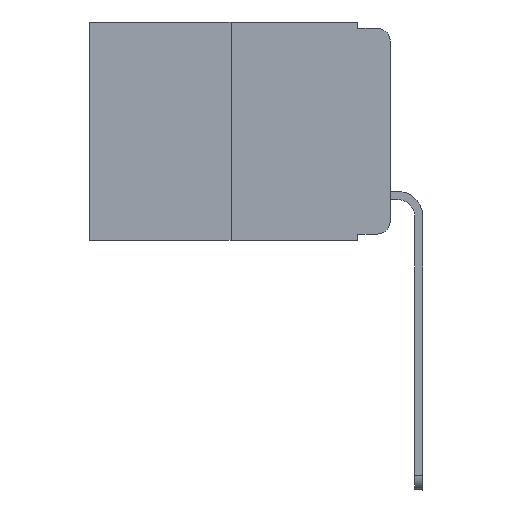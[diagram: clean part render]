
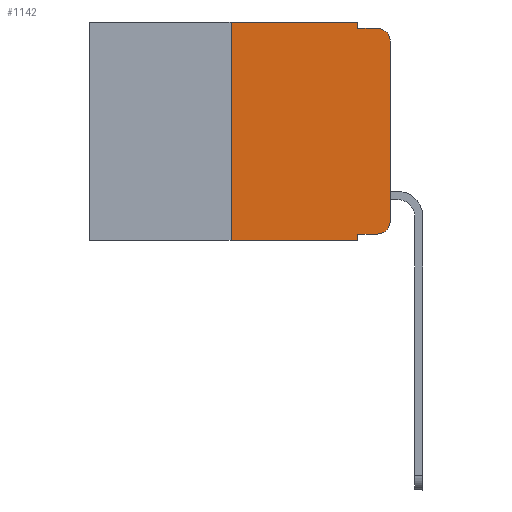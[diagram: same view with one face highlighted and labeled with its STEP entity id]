
A CAD part, left-side view. The second image highlights one B-rep face of the part: STEP entity #1142.
In plain terms, the highlighted planar face has unit normal (-1, 0, 0).
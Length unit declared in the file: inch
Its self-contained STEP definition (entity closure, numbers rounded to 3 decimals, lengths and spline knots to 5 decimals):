
#118 = LINE ( 'NONE', #17399, #14100 ) ;
#137 = CARTESIAN_POINT ( 'NONE',  ( 0., 0.25, 0. ) ) ;
#210 = VECTOR ( 'NONE', #14992, 39.37008 ) ;
#268 = CIRCLE ( 'NONE', #9839, 0.02 ) ;
#355 = DIRECTION ( 'NONE',  ( 0., 0., -1. ) ) ;
#669 = EDGE_CURVE ( 'NONE', #5832, #14060, #118, .T. ) ;
#944 = CARTESIAN_POINT ( 'NONE',  ( 0., 0.25, -0.343 ) ) ;
#1142 = ADVANCED_FACE ( 'NONE', ( #17478 ), #5065, .F. ) ;
#1300 = VERTEX_POINT ( 'NONE', #16242 ) ;
#2220 = CARTESIAN_POINT ( 'NONE',  ( 0., 0.051, 0. ) ) ;
#2387 = ORIENTED_EDGE ( 'NONE', *, *, #20250, .F. ) ;
#3451 = ORIENTED_EDGE ( 'NONE', *, *, #10100, .F. ) ;
#3879 = EDGE_LOOP ( 'NONE', ( #17752, #15207, #17142, #3451, #15063, #2387, #17645, #16792, #17777, #17153 ) ) ;
#3902 = VECTOR ( 'NONE', #18713, 39.37008 ) ;
#3994 = CARTESIAN_POINT ( 'NONE',  ( 0., 0., -0.313 ) ) ;
#4027 = VERTEX_POINT ( 'NONE', #12173 ) ;
#4070 = LINE ( 'NONE', #15347, #5604 ) ;
#4444 = DIRECTION ( 'NONE',  ( -1., 0., 0. ) ) ;
#5065 = PLANE ( 'NONE',  #8002 ) ;
#5604 = VECTOR ( 'NONE', #8839, 39.37008 ) ;
#5832 = VERTEX_POINT ( 'NONE', #19000 ) ;
#6149 = CARTESIAN_POINT ( 'NONE',  ( 0., 0.02, -0.01 ) ) ;
#6307 = EDGE_CURVE ( 'NONE', #10307, #6653, #14230, .T. ) ;
#6369 = CARTESIAN_POINT ( 'NONE',  ( 0., 0., 0. ) ) ;
#6458 = DIRECTION ( 'NONE',  ( 0., 0., 1. ) ) ;
#6544 = DIRECTION ( 'NONE',  ( 0., -1., 0. ) ) ;
#6653 = VERTEX_POINT ( 'NONE', #20296 ) ;
#6785 = AXIS2_PLACEMENT_3D ( 'NONE', #16962, #4444, #19852 ) ;
#6885 = LINE ( 'NONE', #2220, #15857 ) ;
#6969 = VERTEX_POINT ( 'NONE', #7750 ) ;
#6989 = DIRECTION ( 'NONE',  ( -1., 0., 0. ) ) ;
#7430 = VECTOR ( 'NONE', #15981, 39.37008 ) ;
#7750 = CARTESIAN_POINT ( 'NONE',  ( 0., 0.25, 0. ) ) ;
#7893 = EDGE_CURVE ( 'NONE', #6969, #1300, #4070, .T. ) ;
#8002 = AXIS2_PLACEMENT_3D ( 'NONE', #9623, #14178, #19233 ) ;
#8839 = DIRECTION ( 'NONE',  ( 0., -1., 0. ) ) ;
#8868 = EDGE_CURVE ( 'NONE', #11155, #14629, #9200, .T. ) ;
#8897 = EDGE_CURVE ( 'NONE', #11449, #10307, #268, .T. ) ;
#9062 = VECTOR ( 'NONE', #6458, 39.37008 ) ;
#9200 = LINE ( 'NONE', #12411, #3902 ) ;
#9623 = CARTESIAN_POINT ( 'NONE',  ( 0., 0.473, 0. ) ) ;
#9724 = CARTESIAN_POINT ( 'NONE',  ( 0., 0.02, -0.333 ) ) ;
#9839 = AXIS2_PLACEMENT_3D ( 'NONE', #18035, #6989, #14740 ) ;
#10100 = EDGE_CURVE ( 'NONE', #1300, #5832, #11665, .T. ) ;
#10307 = VERTEX_POINT ( 'NONE', #3994 ) ;
#10661 = EDGE_CURVE ( 'NONE', #4027, #14629, #6885, .T. ) ;
#11155 = VERTEX_POINT ( 'NONE', #944 ) ;
#11379 = CARTESIAN_POINT ( 'NONE',  ( 0., 0.051, -0.343 ) ) ;
#11449 = VERTEX_POINT ( 'NONE', #9724 ) ;
#11665 = LINE ( 'NONE', #17952, #12854 ) ;
#11755 = CIRCLE ( 'NONE', #6785, 0.02 ) ;
#12173 = CARTESIAN_POINT ( 'NONE',  ( 0., 0.051, -0.333 ) ) ;
#12411 = CARTESIAN_POINT ( 'NONE',  ( 0., 0.473, -0.343 ) ) ;
#12847 = EDGE_CURVE ( 'NONE', #4027, #11449, #18193, .T. ) ;
#12854 = VECTOR ( 'NONE', #14659, 39.37008 ) ;
#14060 = VERTEX_POINT ( 'NONE', #6149 ) ;
#14100 = VECTOR ( 'NONE', #6544, 39.37008 ) ;
#14178 = DIRECTION ( 'NONE',  ( 1., 0., 0. ) ) ;
#14230 = LINE ( 'NONE', #6369, #7430 ) ;
#14629 = VERTEX_POINT ( 'NONE', #11379 ) ;
#14659 = DIRECTION ( 'NONE',  ( 0., 0., -1. ) ) ;
#14740 = DIRECTION ( 'NONE',  ( 0., 0., -1. ) ) ;
#14877 = EDGE_CURVE ( 'NONE', #6653, #14060, #11755, .T. ) ;
#14992 = DIRECTION ( 'NONE',  ( 0., -1., 0. ) ) ;
#15063 = ORIENTED_EDGE ( 'NONE', *, *, #7893, .F. ) ;
#15207 = ORIENTED_EDGE ( 'NONE', *, *, #14877, .T. ) ;
#15347 = CARTESIAN_POINT ( 'NONE',  ( 0., 0.473, 0. ) ) ;
#15574 = LINE ( 'NONE', #137, #9062 ) ;
#15857 = VECTOR ( 'NONE', #355, 39.37008 ) ;
#15981 = DIRECTION ( 'NONE',  ( 0., 0., 1. ) ) ;
#16242 = CARTESIAN_POINT ( 'NONE',  ( 0., 0.051, 0. ) ) ;
#16792 = ORIENTED_EDGE ( 'NONE', *, *, #10661, .F. ) ;
#16962 = CARTESIAN_POINT ( 'NONE',  ( 0., 0.02, -0.03 ) ) ;
#17142 = ORIENTED_EDGE ( 'NONE', *, *, #669, .F. ) ;
#17153 = ORIENTED_EDGE ( 'NONE', *, *, #8897, .T. ) ;
#17399 = CARTESIAN_POINT ( 'NONE',  ( 0., 0.051, -0.01 ) ) ;
#17478 = FACE_OUTER_BOUND ( 'NONE', #3879, .T. ) ;
#17645 = ORIENTED_EDGE ( 'NONE', *, *, #8868, .T. ) ;
#17752 = ORIENTED_EDGE ( 'NONE', *, *, #6307, .T. ) ;
#17777 = ORIENTED_EDGE ( 'NONE', *, *, #12847, .T. ) ;
#17952 = CARTESIAN_POINT ( 'NONE',  ( 0., 0.051, 0. ) ) ;
#18035 = CARTESIAN_POINT ( 'NONE',  ( 0., 0.02, -0.313 ) ) ;
#18193 = LINE ( 'NONE', #19953, #210 ) ;
#18713 = DIRECTION ( 'NONE',  ( 0., -1., 0. ) ) ;
#19000 = CARTESIAN_POINT ( 'NONE',  ( 0., 0.051, -0.01 ) ) ;
#19233 = DIRECTION ( 'NONE',  ( 0., 0., -1. ) ) ;
#19852 = DIRECTION ( 'NONE',  ( 0., 0., -1. ) ) ;
#19953 = CARTESIAN_POINT ( 'NONE',  ( 0., 0.051, -0.333 ) ) ;
#20250 = EDGE_CURVE ( 'NONE', #11155, #6969, #15574, .T. ) ;
#20296 = CARTESIAN_POINT ( 'NONE',  ( 0., 0., -0.03 ) ) ;
